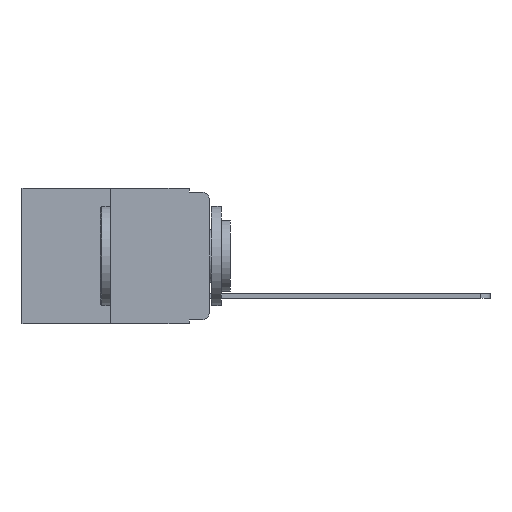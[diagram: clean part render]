
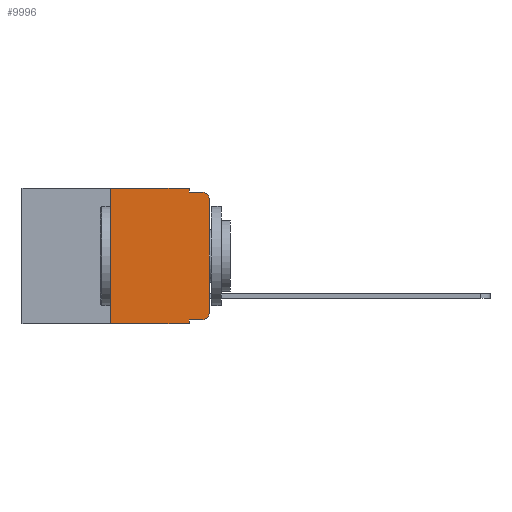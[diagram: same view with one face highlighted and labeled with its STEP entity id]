
A CAD part, left-side view. The second image highlights one B-rep face of the part: STEP entity #9996.
In plain terms, the highlighted planar face has unit normal (-1, 0, 0).
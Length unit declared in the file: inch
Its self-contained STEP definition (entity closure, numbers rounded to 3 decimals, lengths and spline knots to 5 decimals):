
#26 = CARTESIAN_POINT ( 'NONE',  ( 0., 0.02, -0.03 ) ) ;
#463 = LINE ( 'NONE', #10358, #19498 ) ;
#533 = EDGE_CURVE ( 'NONE', #10571, #12834, #1433, .T. ) ;
#700 = EDGE_CURVE ( 'NONE', #9043, #10571, #2237, .T. ) ;
#766 = EDGE_CURVE ( 'NONE', #9043, #12491, #3971, .T. ) ;
#1065 = EDGE_CURVE ( 'NONE', #9007, #7050, #9615, .T. ) ;
#1406 = EDGE_CURVE ( 'NONE', #10533, #10200, #3702, .T. ) ;
#1433 = CIRCLE ( 'NONE', #16290, 0.02 ) ;
#1478 = EDGE_CURVE ( 'NONE', #10200, #6932, #10100, .T. ) ;
#1618 = CARTESIAN_POINT ( 'NONE',  ( 0., 0.02, -0.333 ) ) ;
#1641 = EDGE_CURVE ( 'NONE', #12369, #6932, #14361, .T. ) ;
#1644 = EDGE_CURVE ( 'NONE', #12834, #12369, #6083, .T. ) ;
#1651 = VECTOR ( 'NONE', #5921, 39.37008 ) ;
#1698 = VECTOR ( 'NONE', #17201, 39.37008 ) ;
#1872 = PLANE ( 'NONE',  #5472 ) ;
#2237 = LINE ( 'NONE', #13604, #1698 ) ;
#2794 = CARTESIAN_POINT ( 'NONE',  ( 0., 0.25, 0. ) ) ;
#3185 = ORIENTED_EDGE ( 'NONE', *, *, #700, .T. ) ;
#3469 = EDGE_CURVE ( 'NONE', #9007, #12491, #10008, .T. ) ;
#3503 = DIRECTION ( 'NONE',  ( 1., 0., 0. ) ) ;
#3702 = LINE ( 'NONE', #7840, #15528 ) ;
#3971 = LINE ( 'NONE', #11657, #19626 ) ;
#4655 = DIRECTION ( 'NONE',  ( 0., 0., -1. ) ) ;
#5151 = EDGE_LOOP ( 'NONE', ( #8100, #16233, #9103, #9598, #17567, #5835, #18461, #6862, #3185, #7336 ) ) ;
#5294 = CARTESIAN_POINT ( 'NONE',  ( 0., 0.051, -0.333 ) ) ;
#5472 = AXIS2_PLACEMENT_3D ( 'NONE', #12870, #3503, #14356 ) ;
#5512 = CARTESIAN_POINT ( 'NONE',  ( 0., 0.02, -0.01 ) ) ;
#5683 = CARTESIAN_POINT ( 'NONE',  ( 0., 0.02, -0.313 ) ) ;
#5835 = ORIENTED_EDGE ( 'NONE', *, *, #1065, .F. ) ;
#5862 = EDGE_CURVE ( 'NONE', #7050, #10533, #463, .T. ) ;
#5910 = CARTESIAN_POINT ( 'NONE',  ( 0., 0., -0.313 ) ) ;
#5921 = DIRECTION ( 'NONE',  ( 0., -1., 0. ) ) ;
#6083 = LINE ( 'NONE', #19264, #9836 ) ;
#6402 = DIRECTION ( 'NONE',  ( 0., 0., 1. ) ) ;
#6776 = CARTESIAN_POINT ( 'NONE',  ( 0., 0.473, -0.343 ) ) ;
#6862 = ORIENTED_EDGE ( 'NONE', *, *, #766, .F. ) ;
#6910 = DIRECTION ( 'NONE',  ( -1., 0., 0. ) ) ;
#6932 = VERTEX_POINT ( 'NONE', #5512 ) ;
#7050 = VERTEX_POINT ( 'NONE', #2794 ) ;
#7336 = ORIENTED_EDGE ( 'NONE', *, *, #533, .T. ) ;
#7588 = DIRECTION ( 'NONE',  ( 0., 0., 1. ) ) ;
#7840 = CARTESIAN_POINT ( 'NONE',  ( 0., 0.051, 0. ) ) ;
#8100 = ORIENTED_EDGE ( 'NONE', *, *, #1644, .T. ) ;
#8396 = CARTESIAN_POINT ( 'NONE',  ( 0., 0.051, -0.343 ) ) ;
#9007 = VERTEX_POINT ( 'NONE', #9970 ) ;
#9043 = VERTEX_POINT ( 'NONE', #5294 ) ;
#9103 = ORIENTED_EDGE ( 'NONE', *, *, #1478, .F. ) ;
#9120 = VECTOR ( 'NONE', #6402, 39.37008 ) ;
#9492 = VECTOR ( 'NONE', #15806, 39.37008 ) ;
#9598 = ORIENTED_EDGE ( 'NONE', *, *, #1406, .F. ) ;
#9615 = LINE ( 'NONE', #18555, #9120 ) ;
#9836 = VECTOR ( 'NONE', #7588, 39.37008 ) ;
#9970 = CARTESIAN_POINT ( 'NONE',  ( 0., 0.25, -0.343 ) ) ;
#9996 = ADVANCED_FACE ( 'NONE', ( #17737 ), #1872, .F. ) ;
#10008 = LINE ( 'NONE', #6776, #9492 ) ;
#10100 = LINE ( 'NONE', #14618, #1651 ) ;
#10200 = VERTEX_POINT ( 'NONE', #10292 ) ;
#10292 = CARTESIAN_POINT ( 'NONE',  ( 0., 0.051, -0.01 ) ) ;
#10358 = CARTESIAN_POINT ( 'NONE',  ( 0., 0.473, 0. ) ) ;
#10366 = AXIS2_PLACEMENT_3D ( 'NONE', #26, #13491, #13600 ) ;
#10533 = VERTEX_POINT ( 'NONE', #14076 ) ;
#10571 = VERTEX_POINT ( 'NONE', #1618 ) ;
#11496 = DIRECTION ( 'NONE',  ( 0., 0., -1. ) ) ;
#11657 = CARTESIAN_POINT ( 'NONE',  ( 0., 0.051, 0. ) ) ;
#11693 = DIRECTION ( 'NONE',  ( 0., 0., -1. ) ) ;
#11911 = DIRECTION ( 'NONE',  ( 0., -1., 0. ) ) ;
#12369 = VERTEX_POINT ( 'NONE', #18688 ) ;
#12491 = VERTEX_POINT ( 'NONE', #8396 ) ;
#12834 = VERTEX_POINT ( 'NONE', #5910 ) ;
#12870 = CARTESIAN_POINT ( 'NONE',  ( 0., 0.473, 0. ) ) ;
#13491 = DIRECTION ( 'NONE',  ( -1., 0., 0. ) ) ;
#13600 = DIRECTION ( 'NONE',  ( 0., 0., -1. ) ) ;
#13604 = CARTESIAN_POINT ( 'NONE',  ( 0., 0.051, -0.333 ) ) ;
#14076 = CARTESIAN_POINT ( 'NONE',  ( 0., 0.051, 0. ) ) ;
#14356 = DIRECTION ( 'NONE',  ( 0., 0., -1. ) ) ;
#14361 = CIRCLE ( 'NONE', #10366, 0.02 ) ;
#14618 = CARTESIAN_POINT ( 'NONE',  ( 0., 0.051, -0.01 ) ) ;
#15528 = VECTOR ( 'NONE', #4655, 39.37008 ) ;
#15806 = DIRECTION ( 'NONE',  ( 0., -1., 0. ) ) ;
#16233 = ORIENTED_EDGE ( 'NONE', *, *, #1641, .T. ) ;
#16290 = AXIS2_PLACEMENT_3D ( 'NONE', #5683, #6910, #11496 ) ;
#17201 = DIRECTION ( 'NONE',  ( 0., -1., 0. ) ) ;
#17567 = ORIENTED_EDGE ( 'NONE', *, *, #5862, .F. ) ;
#17737 = FACE_OUTER_BOUND ( 'NONE', #5151, .T. ) ;
#18461 = ORIENTED_EDGE ( 'NONE', *, *, #3469, .T. ) ;
#18555 = CARTESIAN_POINT ( 'NONE',  ( 0., 0.25, 0. ) ) ;
#18688 = CARTESIAN_POINT ( 'NONE',  ( 0., 0., -0.03 ) ) ;
#19264 = CARTESIAN_POINT ( 'NONE',  ( 0., 0., 0. ) ) ;
#19498 = VECTOR ( 'NONE', #11911, 39.37008 ) ;
#19626 = VECTOR ( 'NONE', #11693, 39.37008 ) ;
